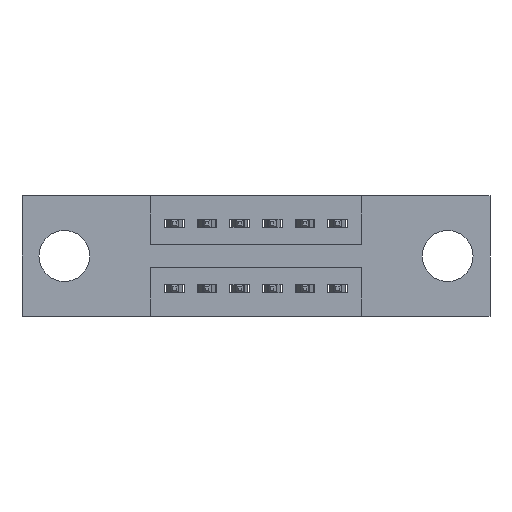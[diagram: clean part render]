
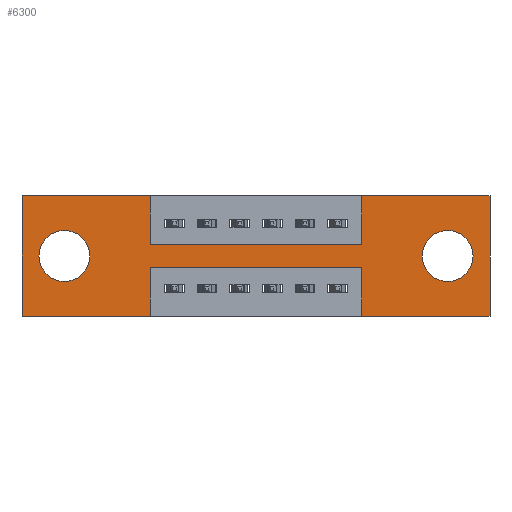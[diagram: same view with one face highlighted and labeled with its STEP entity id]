
A CAD part, front view. The second image highlights one B-rep face of the part: STEP entity #6300.
In plain terms, the highlighted planar face has unit normal (0, -1, 0).
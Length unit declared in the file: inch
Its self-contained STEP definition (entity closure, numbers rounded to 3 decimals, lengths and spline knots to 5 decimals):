
#25 = CIRCLE ( 'NONE', #2988, 0.078 ) ;
#155 = CARTESIAN_POINT ( 'NONE',  ( 0., 0., -0.37 ) ) ;
#277 = CARTESIAN_POINT ( 'NONE',  ( 0.3925, 0., -0.15 ) ) ;
#342 = DIRECTION ( 'NONE',  ( -1., 0., 0. ) ) ;
#478 = CARTESIAN_POINT ( 'NONE',  ( 0.13, 0., -0.263 ) ) ;
#547 = CARTESIAN_POINT ( 'NONE',  ( 0., 0., 0. ) ) ;
#563 = VECTOR ( 'NONE', #9051, 39.37008 ) ;
#612 = VECTOR ( 'NONE', #1938, 39.37008 ) ;
#693 = CARTESIAN_POINT ( 'NONE',  ( 1.0425, 0., -0.37 ) ) ;
#837 = LINE ( 'NONE', #2309, #5199 ) ;
#1094 = CARTESIAN_POINT ( 'NONE',  ( 0.13, 0., -0.107 ) ) ;
#1101 = LINE ( 'NONE', #155, #8822 ) ;
#1180 = VECTOR ( 'NONE', #7815, 39.37008 ) ;
#1185 = EDGE_CURVE ( 'NONE', #3196, #6696, #7023, .T. ) ;
#1191 = DIRECTION ( 'NONE',  ( 1., 0., 0. ) ) ;
#1266 = CARTESIAN_POINT ( 'NONE',  ( 1.305, 0., -0.107 ) ) ;
#1281 = VERTEX_POINT ( 'NONE', #1306 ) ;
#1303 = DIRECTION ( 'NONE',  ( -1., 0., 0. ) ) ;
#1306 = CARTESIAN_POINT ( 'NONE',  ( 1.0425, 0., -0.22 ) ) ;
#1397 = EDGE_LOOP ( 'NONE', ( #2684, #2696 ) ) ;
#1529 = CARTESIAN_POINT ( 'NONE',  ( 0., 0., 0. ) ) ;
#1858 = VERTEX_POINT ( 'NONE', #3031 ) ;
#1893 = DIRECTION ( 'NONE',  ( 0., 0., -1. ) ) ;
#1916 = DIRECTION ( 'NONE',  ( 0., 1., 0. ) ) ;
#1917 = CARTESIAN_POINT ( 'NONE',  ( 1.305, 0., -0.185 ) ) ;
#1938 = DIRECTION ( 'NONE',  ( 0., 0., -1. ) ) ;
#2271 = VERTEX_POINT ( 'NONE', #5076 ) ;
#2309 = CARTESIAN_POINT ( 'NONE',  ( 0., 0., 0. ) ) ;
#2398 = VECTOR ( 'NONE', #1303, 39.37008 ) ;
#2558 = CARTESIAN_POINT ( 'NONE',  ( 1.0425, 0., -0.37 ) ) ;
#2654 = ORIENTED_EDGE ( 'NONE', *, *, #4621, .T. ) ;
#2665 = ORIENTED_EDGE ( 'NONE', *, *, #4822, .T. ) ;
#2682 = FACE_BOUND ( 'NONE', #1397, .T. ) ;
#2684 = ORIENTED_EDGE ( 'NONE', *, *, #3351, .T. ) ;
#2696 = ORIENTED_EDGE ( 'NONE', *, *, #3895, .T. ) ;
#2706 = ORIENTED_EDGE ( 'NONE', *, *, #7589, .F. ) ;
#2752 = ORIENTED_EDGE ( 'NONE', *, *, #3016, .F. ) ;
#2793 = DIRECTION ( 'NONE',  ( 0., 1., 0. ) ) ;
#2804 = ORIENTED_EDGE ( 'NONE', *, *, #6866, .F. ) ;
#2812 = ORIENTED_EDGE ( 'NONE', *, *, #7824, .F. ) ;
#2835 = ORIENTED_EDGE ( 'NONE', *, *, #1185, .F. ) ;
#2854 = ORIENTED_EDGE ( 'NONE', *, *, #9439, .F. ) ;
#2855 = LINE ( 'NONE', #6479, #563 ) ;
#2861 = CARTESIAN_POINT ( 'NONE',  ( 0., 0., 0. ) ) ;
#2862 = ORIENTED_EDGE ( 'NONE', *, *, #9093, .F. ) ;
#2863 = AXIS2_PLACEMENT_3D ( 'NONE', #4508, #4506, #4485 ) ;
#2888 = ORIENTED_EDGE ( 'NONE', *, *, #9240, .F. ) ;
#2915 = ORIENTED_EDGE ( 'NONE', *, *, #9002, .F. ) ;
#2917 = ORIENTED_EDGE ( 'NONE', *, *, #9216, .F. ) ;
#2927 = ORIENTED_EDGE ( 'NONE', *, *, #7943, .F. ) ;
#2959 = ORIENTED_EDGE ( 'NONE', *, *, #4216, .F. ) ;
#2978 = VERTEX_POINT ( 'NONE', #1094 ) ;
#2988 = AXIS2_PLACEMENT_3D ( 'NONE', #1917, #1916, #1893 ) ;
#2991 = VECTOR ( 'NONE', #3111, 39.37008 ) ;
#3016 = EDGE_CURVE ( 'NONE', #1281, #6067, #7002, .T. ) ;
#3031 = CARTESIAN_POINT ( 'NONE',  ( 0.3925, 0., -0.15 ) ) ;
#3111 = DIRECTION ( 'NONE',  ( 0., 0., 1. ) ) ;
#3196 = VERTEX_POINT ( 'NONE', #5173 ) ;
#3201 = LINE ( 'NONE', #2861, #7084 ) ;
#3210 = VERTEX_POINT ( 'NONE', #1529 ) ;
#3351 = EDGE_CURVE ( 'NONE', #2978, #5090, #4886, .T. ) ;
#3516 = DIRECTION ( 'NONE',  ( 0., 0., 1. ) ) ;
#3544 = DIRECTION ( 'NONE',  ( 0., 0., -1. ) ) ;
#3546 = VERTEX_POINT ( 'NONE', #3931 ) ;
#3557 = AXIS2_PLACEMENT_3D ( 'NONE', #7171, #3746, #3516 ) ;
#3651 = DIRECTION ( 'NONE',  ( 1., 0., 0. ) ) ;
#3746 = DIRECTION ( 'NONE',  ( 0., 1., 0. ) ) ;
#3782 = CARTESIAN_POINT ( 'NONE',  ( 0.3925, 0., -0.22 ) ) ;
#3793 = CARTESIAN_POINT ( 'NONE',  ( 0., 0., -0.37 ) ) ;
#3895 = EDGE_CURVE ( 'NONE', #5090, #2978, #9553, .T. ) ;
#3931 = CARTESIAN_POINT ( 'NONE',  ( 1.305, 0., -0.263 ) ) ;
#4044 = VERTEX_POINT ( 'NONE', #693 ) ;
#4216 = EDGE_CURVE ( 'NONE', #6709, #4361, #1101, .T. ) ;
#4271 = LINE ( 'NONE', #5832, #7871 ) ;
#4361 = VERTEX_POINT ( 'NONE', #7663 ) ;
#4410 = VERTEX_POINT ( 'NONE', #7063 ) ;
#4485 = DIRECTION ( 'NONE',  ( 0., 0., -1. ) ) ;
#4506 = DIRECTION ( 'NONE',  ( 0., 1., 0. ) ) ;
#4508 = CARTESIAN_POINT ( 'NONE',  ( 1.305, 0., -0.185 ) ) ;
#4600 = FACE_OUTER_BOUND ( 'NONE', #5186, .T. ) ;
#4621 = EDGE_CURVE ( 'NONE', #6435, #3546, #4635, .T. ) ;
#4635 = CIRCLE ( 'NONE', #2863, 0.078 ) ;
#4775 = EDGE_LOOP ( 'NONE', ( #2654, #2665 ) ) ;
#4822 = EDGE_CURVE ( 'NONE', #3546, #6435, #25, .T. ) ;
#4830 = FACE_BOUND ( 'NONE', #4775, .T. ) ;
#4875 = VECTOR ( 'NONE', #1191, 39.37008 ) ;
#4886 = CIRCLE ( 'NONE', #5043, 0.078 ) ;
#5043 = AXIS2_PLACEMENT_3D ( 'NONE', #7220, #2793, #7044 ) ;
#5076 = CARTESIAN_POINT ( 'NONE',  ( 1.0425, 0., -0.15 ) ) ;
#5090 = VERTEX_POINT ( 'NONE', #478 ) ;
#5122 = LINE ( 'NONE', #547, #2991 ) ;
#5131 = LINE ( 'NONE', #9155, #9580 ) ;
#5173 = CARTESIAN_POINT ( 'NONE',  ( 1.435, 0., 0. ) ) ;
#5186 = EDGE_LOOP ( 'NONE', ( #2706, #2752, #2804, #2812, #2835, #2854, #2862, #2888, #2915, #2917, #2927, #2959 ) ) ;
#5199 = VECTOR ( 'NONE', #7624, 39.37008 ) ;
#5218 = CARTESIAN_POINT ( 'NONE',  ( 1.435, 0., 0. ) ) ;
#5439 = VECTOR ( 'NONE', #5809, 39.37008 ) ;
#5809 = DIRECTION ( 'NONE',  ( -1., 0., 0. ) ) ;
#5832 = CARTESIAN_POINT ( 'NONE',  ( 1.0425, 0., 0. ) ) ;
#5971 = DIRECTION ( 'NONE',  ( 0., 0., -1. ) ) ;
#5976 = AXIS2_PLACEMENT_3D ( 'NONE', #6380, #5993, #5971 ) ;
#5993 = DIRECTION ( 'NONE',  ( 0., -1., 0. ) ) ;
#6067 = VERTEX_POINT ( 'NONE', #3782 ) ;
#6213 = PLANE ( 'NONE',  #5976 ) ;
#6300 = ADVANCED_FACE ( 'NONE', ( #4830, #2682, #4600 ), #6213, .T. ) ;
#6380 = CARTESIAN_POINT ( 'NONE',  ( 0., 0., -0.37 ) ) ;
#6435 = VERTEX_POINT ( 'NONE', #1266 ) ;
#6479 = CARTESIAN_POINT ( 'NONE',  ( 0.3925, 0., 0. ) ) ;
#6617 = CARTESIAN_POINT ( 'NONE',  ( 0.3925, 0., 0. ) ) ;
#6627 = DIRECTION ( 'NONE',  ( 0., 0., 1. ) ) ;
#6696 = VERTEX_POINT ( 'NONE', #8683 ) ;
#6709 = VERTEX_POINT ( 'NONE', #7390 ) ;
#6866 = EDGE_CURVE ( 'NONE', #4044, #1281, #7028, .T. ) ;
#7002 = LINE ( 'NONE', #7312, #5439 ) ;
#7023 = LINE ( 'NONE', #5218, #612 ) ;
#7028 = LINE ( 'NONE', #2558, #1180 ) ;
#7044 = DIRECTION ( 'NONE',  ( 0., 0., 1. ) ) ;
#7063 = CARTESIAN_POINT ( 'NONE',  ( 1.0425, 0., 0. ) ) ;
#7084 = VECTOR ( 'NONE', #3651, 39.37008 ) ;
#7171 = CARTESIAN_POINT ( 'NONE',  ( 0.13, 0., -0.185 ) ) ;
#7220 = CARTESIAN_POINT ( 'NONE',  ( 0.13, 0., -0.185 ) ) ;
#7312 = CARTESIAN_POINT ( 'NONE',  ( 0.3925, 0., -0.22 ) ) ;
#7390 = CARTESIAN_POINT ( 'NONE',  ( 0.3925, 0., -0.37 ) ) ;
#7574 = VERTEX_POINT ( 'NONE', #6617 ) ;
#7589 = EDGE_CURVE ( 'NONE', #6067, #6709, #5131, .T. ) ;
#7624 = DIRECTION ( 'NONE',  ( 1., 0., 0. ) ) ;
#7663 = CARTESIAN_POINT ( 'NONE',  ( 0., 0., -0.37 ) ) ;
#7815 = DIRECTION ( 'NONE',  ( 0., 0., 1. ) ) ;
#7824 = EDGE_CURVE ( 'NONE', #6696, #4044, #8103, .T. ) ;
#7871 = VECTOR ( 'NONE', #6627, 39.37008 ) ;
#7943 = EDGE_CURVE ( 'NONE', #4361, #3210, #5122, .T. ) ;
#8103 = LINE ( 'NONE', #3793, #2398 ) ;
#8683 = CARTESIAN_POINT ( 'NONE',  ( 1.435, 0., -0.37 ) ) ;
#8752 = LINE ( 'NONE', #277, #4875 ) ;
#8822 = VECTOR ( 'NONE', #342, 39.37008 ) ;
#9002 = EDGE_CURVE ( 'NONE', #7574, #1858, #2855, .T. ) ;
#9051 = DIRECTION ( 'NONE',  ( 0., 0., -1. ) ) ;
#9093 = EDGE_CURVE ( 'NONE', #2271, #4410, #4271, .T. ) ;
#9155 = CARTESIAN_POINT ( 'NONE',  ( 0.3925, 0., -0.37 ) ) ;
#9216 = EDGE_CURVE ( 'NONE', #3210, #7574, #3201, .T. ) ;
#9240 = EDGE_CURVE ( 'NONE', #1858, #2271, #8752, .T. ) ;
#9439 = EDGE_CURVE ( 'NONE', #4410, #3196, #837, .T. ) ;
#9553 = CIRCLE ( 'NONE', #3557, 0.078 ) ;
#9580 = VECTOR ( 'NONE', #3544, 39.37008 ) ;
